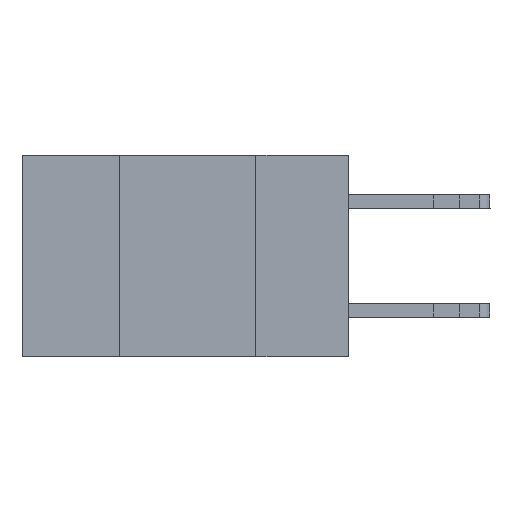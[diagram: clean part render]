
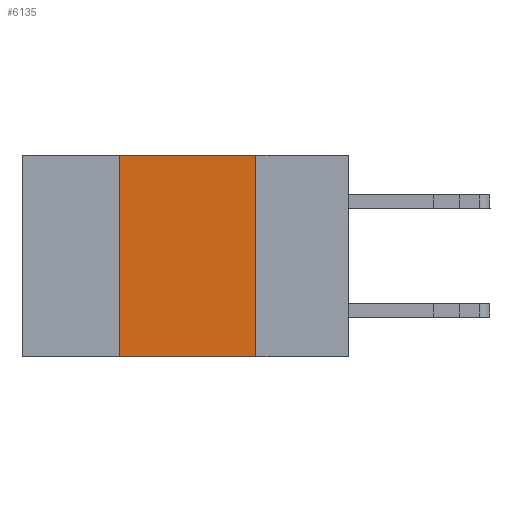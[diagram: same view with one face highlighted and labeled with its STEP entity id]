
A CAD part, left-side view. The second image highlights one B-rep face of the part: STEP entity #6135.
In plain terms, the highlighted planar face has unit normal (-1, 0, 0).
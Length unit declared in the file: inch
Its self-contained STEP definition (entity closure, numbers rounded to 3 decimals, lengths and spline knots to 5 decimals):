
#322 = DIRECTION ( 'NONE',  ( 0., 0., -1. ) ) ;
#495 = VECTOR ( 'NONE', #674, 39.37008 ) ;
#674 = DIRECTION ( 'NONE',  ( 0., 0., 1. ) ) ;
#707 = VERTEX_POINT ( 'NONE', #12492 ) ;
#730 = DIRECTION ( 'NONE',  ( 0., -1., 0. ) ) ;
#968 = LINE ( 'NONE', #14520, #17655 ) ;
#1390 = CARTESIAN_POINT ( 'NONE',  ( 0., 0.42, -0.37 ) ) ;
#1563 = VECTOR ( 'NONE', #3904, 39.37008 ) ;
#2250 = EDGE_LOOP ( 'NONE', ( #16287, #2682, #17348, #21708 ) ) ;
#2575 = EDGE_CURVE ( 'NONE', #15942, #707, #11691, .T. ) ;
#2682 = ORIENTED_EDGE ( 'NONE', *, *, #14900, .F. ) ;
#3904 = DIRECTION ( 'NONE',  ( 0., -1., 0. ) ) ;
#4957 = CARTESIAN_POINT ( 'NONE',  ( 0., 0.42, 0. ) ) ;
#6065 = LINE ( 'NONE', #18119, #1563 ) ;
#6135 = ADVANCED_FACE ( 'NONE', ( #12884 ), #9452, .F. ) ;
#6333 = DIRECTION ( 'NONE',  ( 0., 0., -1. ) ) ;
#6659 = AXIS2_PLACEMENT_3D ( 'NONE', #12993, #7404, #322 ) ;
#7404 = DIRECTION ( 'NONE',  ( 1., 0., 0. ) ) ;
#9452 = PLANE ( 'NONE',  #6659 ) ;
#10254 = EDGE_CURVE ( 'NONE', #16547, #707, #6065, .T. ) ;
#10812 = VERTEX_POINT ( 'NONE', #4957 ) ;
#11032 = CARTESIAN_POINT ( 'NONE',  ( 0., 0.17, 0. ) ) ;
#11521 = CARTESIAN_POINT ( 'NONE',  ( 0., 0.42, -0.37 ) ) ;
#11691 = LINE ( 'NONE', #18605, #17526 ) ;
#12492 = CARTESIAN_POINT ( 'NONE',  ( 0., 0.17, -0.37 ) ) ;
#12538 = EDGE_CURVE ( 'NONE', #16547, #10812, #19926, .T. ) ;
#12884 = FACE_OUTER_BOUND ( 'NONE', #2250, .T. ) ;
#12993 = CARTESIAN_POINT ( 'NONE',  ( 0., 0.6, 0. ) ) ;
#14520 = CARTESIAN_POINT ( 'NONE',  ( 0., 0.6, 0. ) ) ;
#14900 = EDGE_CURVE ( 'NONE', #10812, #15942, #968, .T. ) ;
#15942 = VERTEX_POINT ( 'NONE', #11032 ) ;
#16287 = ORIENTED_EDGE ( 'NONE', *, *, #2575, .F. ) ;
#16547 = VERTEX_POINT ( 'NONE', #1390 ) ;
#17348 = ORIENTED_EDGE ( 'NONE', *, *, #12538, .F. ) ;
#17526 = VECTOR ( 'NONE', #6333, 39.37008 ) ;
#17655 = VECTOR ( 'NONE', #730, 39.37008 ) ;
#18119 = CARTESIAN_POINT ( 'NONE',  ( 0., 0.6, -0.37 ) ) ;
#18605 = CARTESIAN_POINT ( 'NONE',  ( 0., 0.17, -0.37 ) ) ;
#19926 = LINE ( 'NONE', #11521, #495 ) ;
#21708 = ORIENTED_EDGE ( 'NONE', *, *, #10254, .T. ) ;
